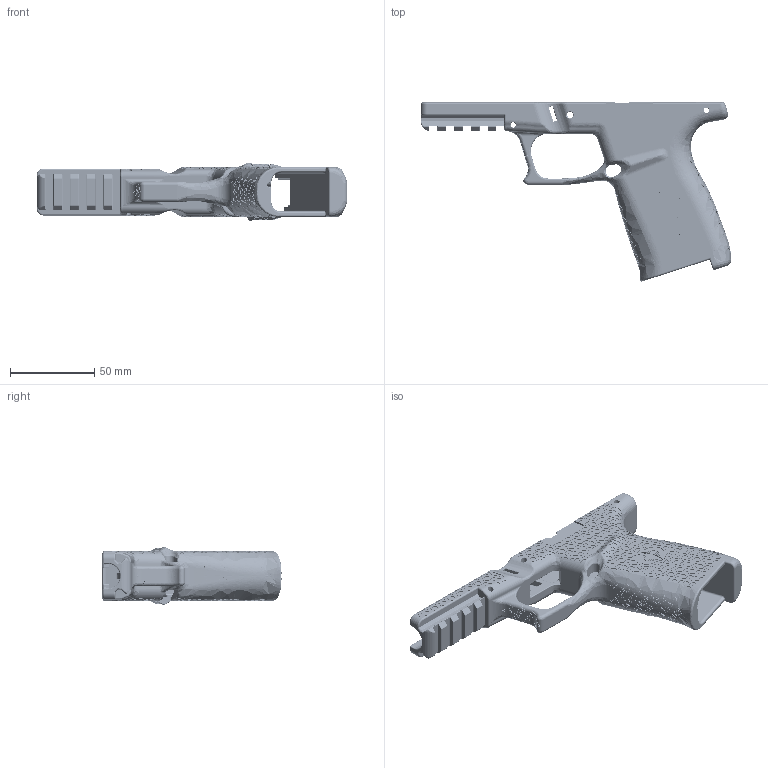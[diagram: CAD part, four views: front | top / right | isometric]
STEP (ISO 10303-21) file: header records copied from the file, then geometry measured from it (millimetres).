
FILE_DESCRIPTION(/* description */ (''),/* implementation_level */ '2;1');
FILE_NAME(/* name */ 'SD40_Carbon Cobra_v0.6_011522.stp',/* time_stamp */ '2022-01-15T17:22:54-05:00',/* author */ (''),/* organization */ (''),/* preprocessor_version */ 'ST-DEVELOPER v16.7',/* originating_system */ 'SIEMENS PLM Software NX 1899',/* authorisation */ '');
FILE_SCHEMA (('AUTOMOTIVE_DESIGN { 1 0 10303 214 3 1 1 1 }'));
Products named in the file (1): tyle19C8C564rekf
Bounding box: 183.88 x 105.98 x 34.01 mm (x, y, z)
Volume: 93449.8 mm3; surface area: 51302.7 mm2
Topology: 1 solids, 1 shells, 12331 faces, 31653 edges, 20640 vertices
Faces by surface type: plane 6571, extrusion 2504, bspline 1508, cylinder 1381, torus 302, cone 43, sphere 22
Full cylindrical faces by diameter (mm): 2.159 x1, 2.5 x1, 3.175 x2, 3.3 x2, 3.6 x2
Entity records: 583020 total; most frequent: CARTESIAN_POINT 316160, ORIENTED_EDGE 63100, DIRECTION 38576, EDGE_CURVE 31550, VERTEX_POINT 20631, B_SPLINE_CURVE_WITH_KNOTS 17340, VECTOR 16356, LINE 13852
